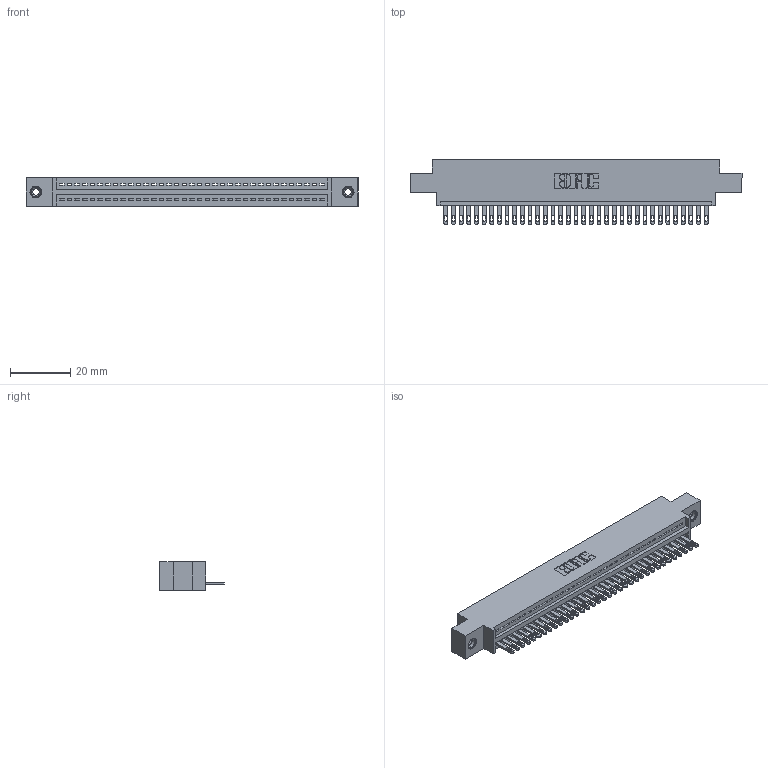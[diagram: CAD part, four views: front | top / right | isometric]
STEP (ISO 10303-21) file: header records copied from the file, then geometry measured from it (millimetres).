
FILE_DESCRIPTION (( 'STEP AP203' ), '1' );
FILE_NAME ('895-035-500-608.STEP', '2020-09-25T22:26:39', ( '' ), ( '' ), 'SwSTEP 2.0', 'SolidWorks 2020', '' );
FILE_SCHEMA (( 'CONFIG_CONTROL_DESIGN' ));
Length unit declared in the file: inch
Products named in the file (4): 345-292-001_345-293-100; 895-035-500-608; 345-250-001_345-250-003-102; 845 Part_0.170 Offset - 0.156 Dia-TI
Assembly tree (38 placements, depth 2):
  895-035-500-608
    845 Part_0.170 Offset - 0.156 Dia-TI
    345-292-001_345-293-100  x35
    345-250-001_345-250-003-102  x2
Bounding box: 110.11 x 21.51 x 9.4 mm (x, y, z)
Volume: 10302.7 mm3; surface area: 13820.5 mm2
Topology: 38 solids, 38 shells, 2080 faces, 6369 edges, 4238 vertices
Faces by surface type: plane 1306, cylinder 758, cone 12, torus 4
Entity records: 28532 total; most frequent: CARTESIAN_POINT 4924, ORIENTED_EDGE 4886, DIRECTION 4339, EDGE_CURVE 2443, LINE 2147, VECTOR 2147, VERTEX_POINT 1624, AXIS2_PLACEMENT_3D 1096
